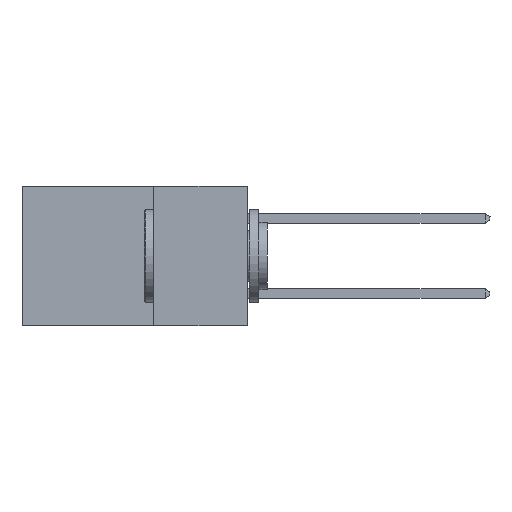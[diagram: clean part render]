
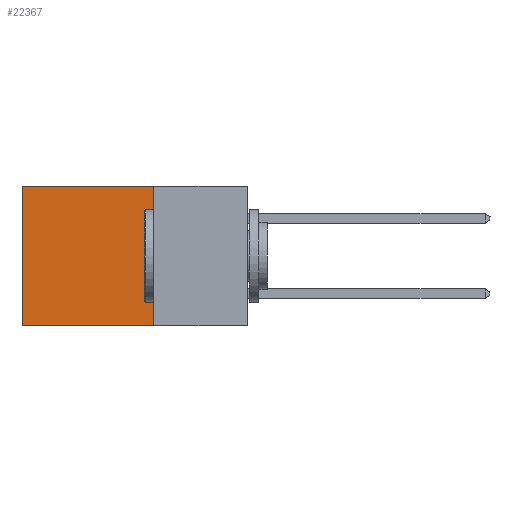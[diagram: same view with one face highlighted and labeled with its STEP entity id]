
A CAD part, left-side view. The second image highlights one B-rep face of the part: STEP entity #22367.
In plain terms, the highlighted planar face has unit normal (-1, 0, 0).
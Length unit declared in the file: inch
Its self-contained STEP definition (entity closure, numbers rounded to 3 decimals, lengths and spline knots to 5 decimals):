
#446 = VERTEX_POINT ( 'NONE', #6623 ) ;
#708 = AXIS2_PLACEMENT_3D ( 'NONE', #13744, #16205, #1362 ) ;
#975 = EDGE_CURVE ( 'NONE', #24304, #14415, #16705, .T. ) ;
#1362 = DIRECTION ( 'NONE',  ( 0., 0., -1. ) ) ;
#1382 = CARTESIAN_POINT ( 'NONE',  ( 0.298, 0.25, -0.37 ) ) ;
#1800 = DIRECTION ( 'NONE',  ( 0., 0., -1. ) ) ;
#1998 = DIRECTION ( 'NONE',  ( 0., 0., -1. ) ) ;
#3470 = VECTOR ( 'NONE', #21578, 39.37008 ) ;
#3728 = EDGE_LOOP ( 'NONE', ( #25778, #4497, #22037, #26518 ) ) ;
#4497 = ORIENTED_EDGE ( 'NONE', *, *, #8964, .F. ) ;
#5025 = LINE ( 'NONE', #19187, #10903 ) ;
#6623 = CARTESIAN_POINT ( 'NONE',  ( 0.298, 0.6, -0.37 ) ) ;
#8697 = PLANE ( 'NONE',  #708 ) ;
#8964 = EDGE_CURVE ( 'NONE', #29977, #446, #14329, .T. ) ;
#10164 = VECTOR ( 'NONE', #1998, 39.37008 ) ;
#10675 = CARTESIAN_POINT ( 'NONE',  ( 0.298, 0.25, -0.37 ) ) ;
#10903 = VECTOR ( 'NONE', #1800, 39.37008 ) ;
#12339 = CARTESIAN_POINT ( 'NONE',  ( 0.298, 0.25, 0. ) ) ;
#13552 = VECTOR ( 'NONE', #28529, 39.37008 ) ;
#13744 = CARTESIAN_POINT ( 'NONE',  ( 0.298, 0.25, 0. ) ) ;
#14023 = CARTESIAN_POINT ( 'NONE',  ( 0.298, 0.25, 0. ) ) ;
#14329 = LINE ( 'NONE', #1382, #13552 ) ;
#14415 = VERTEX_POINT ( 'NONE', #28297 ) ;
#16205 = DIRECTION ( 'NONE',  ( 1., 0., 0. ) ) ;
#16705 = LINE ( 'NONE', #14023, #3470 ) ;
#19187 = CARTESIAN_POINT ( 'NONE',  ( 0.298, 0.6, 0. ) ) ;
#21578 = DIRECTION ( 'NONE',  ( 0., 1., 0. ) ) ;
#22037 = ORIENTED_EDGE ( 'NONE', *, *, #24731, .F. ) ;
#22367 = ADVANCED_FACE ( 'NONE', ( #26953 ), #8697, .F. ) ;
#24304 = VERTEX_POINT ( 'NONE', #12339 ) ;
#24333 = CARTESIAN_POINT ( 'NONE',  ( 0.298, 0.25, 0. ) ) ;
#24731 = EDGE_CURVE ( 'NONE', #24304, #29977, #29085, .T. ) ;
#25778 = ORIENTED_EDGE ( 'NONE', *, *, #27064, .T. ) ;
#26518 = ORIENTED_EDGE ( 'NONE', *, *, #975, .T. ) ;
#26953 = FACE_OUTER_BOUND ( 'NONE', #3728, .T. ) ;
#27064 = EDGE_CURVE ( 'NONE', #14415, #446, #5025, .T. ) ;
#28297 = CARTESIAN_POINT ( 'NONE',  ( 0.298, 0.6, 0. ) ) ;
#28529 = DIRECTION ( 'NONE',  ( 0., 1., 0. ) ) ;
#29085 = LINE ( 'NONE', #24333, #10164 ) ;
#29977 = VERTEX_POINT ( 'NONE', #10675 ) ;
